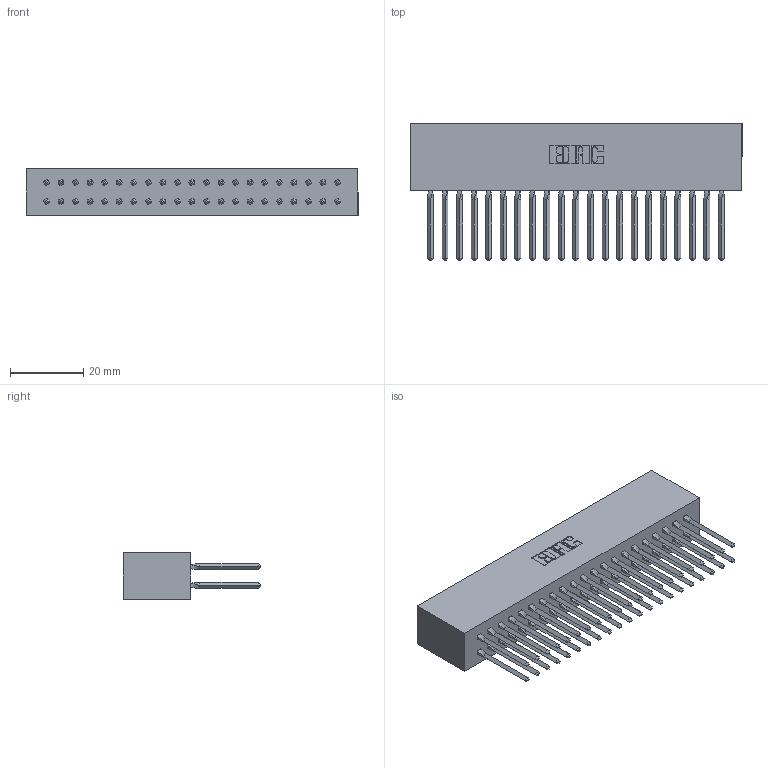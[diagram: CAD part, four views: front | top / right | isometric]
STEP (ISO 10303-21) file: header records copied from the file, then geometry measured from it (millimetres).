
FILE_DESCRIPTION (( 'STEP AP203' ), '1' );
FILE_NAME ('317-042-540-801.STEP', '2020-02-28T01:18:13', ( '' ), ( '' ), 'SwSTEP 2.0', 'SolidWorks 2016', '' );
FILE_SCHEMA (( 'CONFIG_CONTROL_DESIGN' ));
Length unit declared in the file: inch
Products named in the file (3): 317 Part_Lugless; 317-290-001_540; 317-042-540-801
Assembly tree (43 placements, depth 2):
  317-042-540-801
    317 Part_Lugless
    317-290-001_540  x42
Bounding box: 90.42 x 37.34 x 12.7 mm (x, y, z)
Volume: 16259.5 mm3; surface area: 23704.9 mm2
Topology: 43 solids, 43 shells, 3828 faces, 10613 edges, 6836 vertices
Faces by surface type: plane 3116, cylinder 544, bspline 168
Entity records: 32876 total; most frequent: CARTESIAN_POINT 6147, ORIENTED_EDGE 5646, DIRECTION 4705, EDGE_CURVE 2823, LINE 2575, VECTOR 2575, VERTEX_POINT 1875, AXIS2_PLACEMENT_3D 1065
